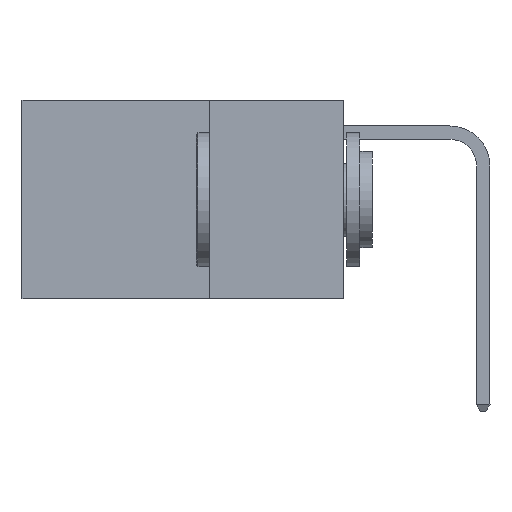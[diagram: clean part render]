
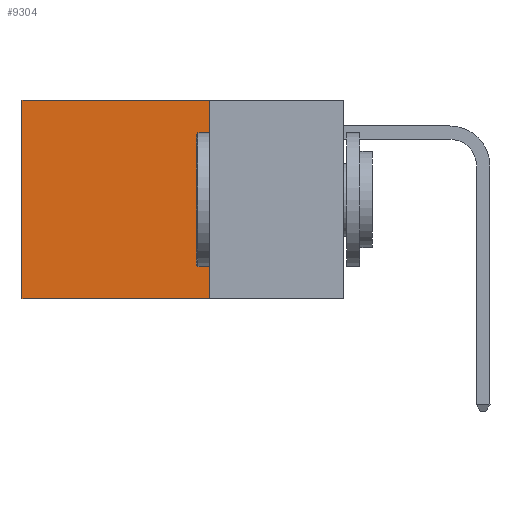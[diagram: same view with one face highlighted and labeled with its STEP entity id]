
A CAD part, left-side view. The second image highlights one B-rep face of the part: STEP entity #9304.
In plain terms, the highlighted planar face has unit normal (-1, 0, 0).
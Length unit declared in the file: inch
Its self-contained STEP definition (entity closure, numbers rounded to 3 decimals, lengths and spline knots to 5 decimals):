
#223 = DIRECTION ( 'NONE',  ( 0., 0., -1. ) ) ;
#604 = CARTESIAN_POINT ( 'NONE',  ( 0.2625, 0.25, 0. ) ) ;
#652 = FACE_OUTER_BOUND ( 'NONE', #10285, .T. ) ;
#1457 = VERTEX_POINT ( 'NONE', #4561 ) ;
#1770 = DIRECTION ( 'NONE',  ( 0., 1., 0. ) ) ;
#1831 = CARTESIAN_POINT ( 'NONE',  ( 0.2625, 0.25, -0.37 ) ) ;
#2103 = AXIS2_PLACEMENT_3D ( 'NONE', #17379, #17219, #17193 ) ;
#4098 = ORIENTED_EDGE ( 'NONE', *, *, #12510, .F. ) ;
#4105 = VERTEX_POINT ( 'NONE', #20501 ) ;
#4561 = CARTESIAN_POINT ( 'NONE',  ( 0.2625, 0.6, -0.37 ) ) ;
#5428 = VECTOR ( 'NONE', #1770, 39.37008 ) ;
#5746 = CARTESIAN_POINT ( 'NONE',  ( 0.2625, 0.25, -0.37 ) ) ;
#6096 = VECTOR ( 'NONE', #8917, 39.37008 ) ;
#6442 = VECTOR ( 'NONE', #12959, 39.37008 ) ;
#8836 = CARTESIAN_POINT ( 'NONE',  ( 0.2625, 0.6, 0. ) ) ;
#8917 = DIRECTION ( 'NONE',  ( 0., 0., -1. ) ) ;
#9304 = ADVANCED_FACE ( 'NONE', ( #652 ), #17459, .F. ) ;
#9880 = EDGE_CURVE ( 'NONE', #4105, #1457, #10198, .T. ) ;
#10198 = LINE ( 'NONE', #8836, #6096 ) ;
#10285 = EDGE_LOOP ( 'NONE', ( #18885, #4098, #16369, #12929 ) ) ;
#11148 = VECTOR ( 'NONE', #223, 39.37008 ) ;
#11686 = LINE ( 'NONE', #21033, #11148 ) ;
#12510 = EDGE_CURVE ( 'NONE', #15540, #1457, #19294, .T. ) ;
#12512 = CARTESIAN_POINT ( 'NONE',  ( 0.2625, 0.25, 0. ) ) ;
#12929 = ORIENTED_EDGE ( 'NONE', *, *, #15062, .T. ) ;
#12959 = DIRECTION ( 'NONE',  ( 0., 1., 0. ) ) ;
#15062 = EDGE_CURVE ( 'NONE', #22445, #4105, #15721, .T. ) ;
#15540 = VERTEX_POINT ( 'NONE', #5746 ) ;
#15721 = LINE ( 'NONE', #12512, #6442 ) ;
#16369 = ORIENTED_EDGE ( 'NONE', *, *, #18165, .F. ) ;
#17193 = DIRECTION ( 'NONE',  ( 0., 0., -1. ) ) ;
#17219 = DIRECTION ( 'NONE',  ( 1., 0., 0. ) ) ;
#17379 = CARTESIAN_POINT ( 'NONE',  ( 0.2625, 0.25, 0. ) ) ;
#17459 = PLANE ( 'NONE',  #2103 ) ;
#18165 = EDGE_CURVE ( 'NONE', #22445, #15540, #11686, .T. ) ;
#18885 = ORIENTED_EDGE ( 'NONE', *, *, #9880, .T. ) ;
#19294 = LINE ( 'NONE', #1831, #5428 ) ;
#20501 = CARTESIAN_POINT ( 'NONE',  ( 0.2625, 0.6, 0. ) ) ;
#21033 = CARTESIAN_POINT ( 'NONE',  ( 0.2625, 0.25, 0. ) ) ;
#22445 = VERTEX_POINT ( 'NONE', #604 ) ;
